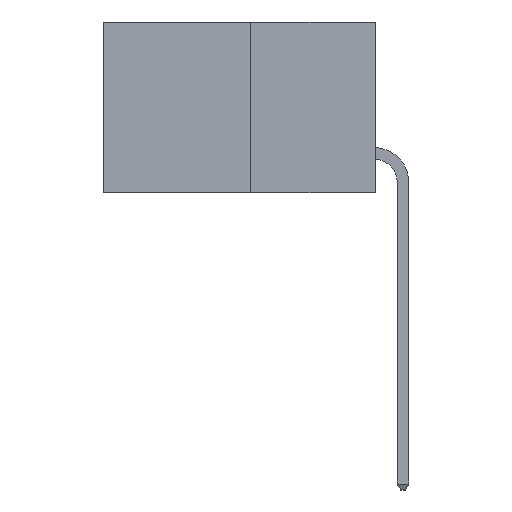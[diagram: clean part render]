
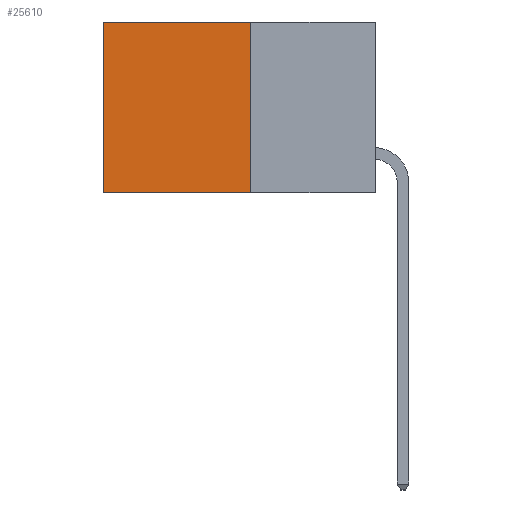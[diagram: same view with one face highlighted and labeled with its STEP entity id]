
A CAD part, left-side view. The second image highlights one B-rep face of the part: STEP entity #25610.
In plain terms, the highlighted planar face has unit normal (-1, 0, 0).
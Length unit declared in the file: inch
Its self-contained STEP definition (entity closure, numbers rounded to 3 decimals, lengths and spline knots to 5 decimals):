
#189 = VERTEX_POINT ( 'NONE', #24651 ) ;
#497 = CARTESIAN_POINT ( 'NONE',  ( 0.277, 0.27, 0. ) ) ;
#1198 = DIRECTION ( 'NONE',  ( 0., 0., -1. ) ) ;
#1925 = VERTEX_POINT ( 'NONE', #19300 ) ;
#2269 = FACE_OUTER_BOUND ( 'NONE', #14057, .T. ) ;
#2958 = VECTOR ( 'NONE', #22744, 39.37008 ) ;
#3495 = VECTOR ( 'NONE', #5408, 39.37008 ) ;
#4028 = CARTESIAN_POINT ( 'NONE',  ( 0.277, 0.27, -0.37 ) ) ;
#5408 = DIRECTION ( 'NONE',  ( 0., 0., -1. ) ) ;
#6204 = EDGE_CURVE ( 'NONE', #24718, #1925, #11831, .T. ) ;
#6373 = CARTESIAN_POINT ( 'NONE',  ( 0.277, 0.27, -0.37 ) ) ;
#7504 = ORIENTED_EDGE ( 'NONE', *, *, #12542, .T. ) ;
#8875 = ORIENTED_EDGE ( 'NONE', *, *, #10405, .F. ) ;
#9201 = LINE ( 'NONE', #6373, #2958 ) ;
#10314 = AXIS2_PLACEMENT_3D ( 'NONE', #13606, #13704, #1198 ) ;
#10405 = EDGE_CURVE ( 'NONE', #24718, #189, #9201, .T. ) ;
#10554 = CARTESIAN_POINT ( 'NONE',  ( 0.277, 0.59, -0.37 ) ) ;
#11603 = PLANE ( 'NONE',  #10314 ) ;
#11831 = LINE ( 'NONE', #24249, #21987 ) ;
#12403 = DIRECTION ( 'NONE',  ( 0., 1., 0. ) ) ;
#12542 = EDGE_CURVE ( 'NONE', #1925, #18088, #19926, .T. ) ;
#12785 = EDGE_CURVE ( 'NONE', #189, #18088, #23708, .T. ) ;
#13606 = CARTESIAN_POINT ( 'NONE',  ( 0.277, 0.27, -0.37 ) ) ;
#13608 = VECTOR ( 'NONE', #12403, 39.37008 ) ;
#13704 = DIRECTION ( 'NONE',  ( 1., 0., 0. ) ) ;
#14057 = EDGE_LOOP ( 'NONE', ( #7504, #23530, #8875, #18598 ) ) ;
#18088 = VERTEX_POINT ( 'NONE', #10554 ) ;
#18598 = ORIENTED_EDGE ( 'NONE', *, *, #6204, .T. ) ;
#19300 = CARTESIAN_POINT ( 'NONE',  ( 0.277, 0.59, 0. ) ) ;
#19780 = CARTESIAN_POINT ( 'NONE',  ( 0.277, 0.59, -0.37 ) ) ;
#19926 = LINE ( 'NONE', #19780, #3495 ) ;
#21987 = VECTOR ( 'NONE', #23523, 39.37008 ) ;
#22744 = DIRECTION ( 'NONE',  ( 0., 0., -1. ) ) ;
#23523 = DIRECTION ( 'NONE',  ( 0., 1., 0. ) ) ;
#23530 = ORIENTED_EDGE ( 'NONE', *, *, #12785, .F. ) ;
#23708 = LINE ( 'NONE', #4028, #13608 ) ;
#24249 = CARTESIAN_POINT ( 'NONE',  ( 0.277, 0.27, 0. ) ) ;
#24651 = CARTESIAN_POINT ( 'NONE',  ( 0.277, 0.27, -0.37 ) ) ;
#24718 = VERTEX_POINT ( 'NONE', #497 ) ;
#25610 = ADVANCED_FACE ( 'NONE', ( #2269 ), #11603, .F. ) ;
